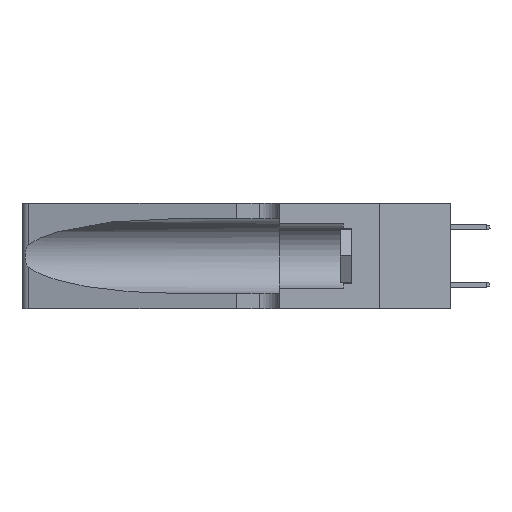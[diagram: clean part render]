
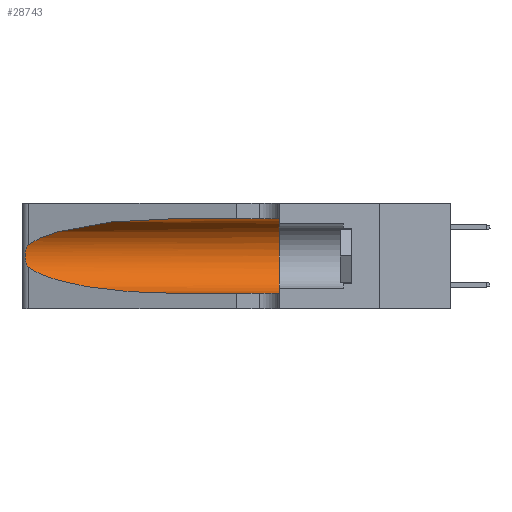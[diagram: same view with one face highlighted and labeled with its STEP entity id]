
A CAD part, left-side view. The second image highlights one B-rep face of the part: STEP entity #28743.
In plain terms, the highlighted cylindrical face has radius 3.308 mm (diameter 6.617 mm), a partial arc.
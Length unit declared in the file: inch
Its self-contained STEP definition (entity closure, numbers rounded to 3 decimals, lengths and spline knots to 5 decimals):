
#1477 = CARTESIAN_POINT ( 'NONE',  ( 0.25854, 1.2359, 0.20912 ) ) ;
#1985 = ORIENTED_EDGE ( 'NONE', *, *, #18966, .F. ) ;
#2399 = VERTEX_POINT ( 'NONE', #12697 ) ;
#2435 = CARTESIAN_POINT ( 'NONE',  ( 0.25487, 1.22718, 0.14631 ) ) ;
#2916 = DIRECTION ( 'NONE',  ( 0., 0., 1. ) ) ;
#3120 = CARTESIAN_POINT ( 'NONE',  ( 0.18966, 0.96281, 0.05475 ) ) ;
#3966 = EDGE_CURVE ( 'NONE', #5168, #22047, #23869, .T. ) ;
#4145 = DIRECTION ( 'NONE',  ( 0., -1., 0. ) ) ;
#5168 = VERTEX_POINT ( 'NONE', #2435 ) ;
#6362 = CARTESIAN_POINT ( 'NONE',  ( 0.18966, 0.96281, 0.31525 ) ) ;
#6592 = CARTESIAN_POINT ( 'NONE',  ( 0.25487, 1.22718, 0.22369 ) ) ;
#6700 = B_SPLINE_CURVE_WITH_KNOTS ( 'NONE', 3,
 ( #29858, #33833, #26591, #15819, #1477, #12050, #41559, #40862, #19999, #26364, #40637, #23302, #19769, #19315 ),
 .UNSPECIFIED., .F., .F.,
 ( 4, 2, 2, 2, 2, 2, 4 ),
 ( 0., 0.00027, 0.00053, 0.00107, 0.0016, 0.00187, 0.00214 ),
 .UNSPECIFIED. ) ;
#7445 = CARTESIAN_POINT ( 'NONE',  ( 0.1305, 1.61858, 0.31525 ) ) ;
#8792 = ORIENTED_EDGE ( 'NONE', *, *, #20589, .T. ) ;
#9802 = CIRCLE ( 'NONE', #37466, 0.13025 ) ;
#10226 = VERTEX_POINT ( 'NONE', #25016 ) ;
#11495 = EDGE_CURVE ( 'NONE', #39197, #2399, #28387, .T. ) ;
#12050 = CARTESIAN_POINT ( 'NONE',  ( 0.26018, 1.23835, 0.19895 ) ) ;
#12697 = CARTESIAN_POINT ( 'NONE',  ( 0.25487, 1.22718, 0.22369 ) ) ;
#13379 = CARTESIAN_POINT ( 'NONE',  ( 0.1305, 0.72297, 0.31525 ) ) ;
#13458 = CARTESIAN_POINT ( 'NONE',  ( 0.1305, 1.61858, 0.185 ) ) ;
#14598 = CARTESIAN_POINT ( 'NONE',  ( 0.1305, 0.72297, 0.05475 ) ) ;
#15301 = ORIENTED_EDGE ( 'NONE', *, *, #45141, .T. ) ;
#15819 = CARTESIAN_POINT ( 'NONE',  ( 0.25787, 1.23484, 0.2124 ) ) ;
#15923 = CARTESIAN_POINT ( 'NONE',  ( 0.1305, 0.35, 0.31525 ) ) ;
#16565 = ORIENTED_EDGE ( 'NONE', *, *, #11495, .T. ) ;
#16692 = ORIENTED_EDGE ( 'NONE', *, *, #3966, .T. ) ;
#17470 = DIRECTION ( 'NONE',  ( 0., 0., -1. ) ) ;
#17496 = ORIENTED_EDGE ( 'NONE', *, *, #27423, .F. ) ;
#18966 = EDGE_CURVE ( 'NONE', #39197, #25622, #22671, .T. ) ;
#19315 = CARTESIAN_POINT ( 'NONE',  ( 0.25487, 1.22718, 0.14631 ) ) ;
#19769 = CARTESIAN_POINT ( 'NONE',  ( 0.25555, 1.22993, 0.14849 ) ) ;
#19999 = CARTESIAN_POINT ( 'NONE',  ( 0.26017, 1.23833, 0.17102 ) ) ;
#20381 = AXIS2_PLACEMENT_3D ( 'NONE', #13458, #27777, #17470 ) ;
#20589 = EDGE_CURVE ( 'NONE', #2399, #5168, #6700, .T. ) ;
#22047 = VERTEX_POINT ( 'NONE', #37639 ) ;
#22671 = LINE ( 'NONE', #7445, #32550 ) ;
#23302 = CARTESIAN_POINT ( 'NONE',  ( 0.25639, 1.23186, 0.15144 ) ) ;
#23869 =( BOUNDED_CURVE ( )  B_SPLINE_CURVE ( 3, ( #25375, #32395, #3120, #14598 ),
 .UNSPECIFIED., .F., .T. ) 
 B_SPLINE_CURVE_WITH_KNOTS ( ( 4, 4 ),
 ( 3.44316, 4.71239 ),
 .UNSPECIFIED. ) 
 CURVE ( )  GEOMETRIC_REPRESENTATION_ITEM ( )  RATIONAL_B_SPLINE_CURVE ( ( 1., 0.87, 0.87, 1. ) ) 
 REPRESENTATION_ITEM ( '' )  );
#24488 = FACE_OUTER_BOUND ( 'NONE', #28070, .T. ) ;
#25016 = CARTESIAN_POINT ( 'NONE',  ( 0.1305, 0.35, 0.05475 ) ) ;
#25375 = CARTESIAN_POINT ( 'NONE',  ( 0.25487, 1.22718, 0.14631 ) ) ;
#25622 = VERTEX_POINT ( 'NONE', #15923 ) ;
#25925 = DIRECTION ( 'NONE',  ( 0., -1., 0. ) ) ;
#26364 = CARTESIAN_POINT ( 'NONE',  ( 0.25856, 1.23593, 0.16098 ) ) ;
#26591 = CARTESIAN_POINT ( 'NONE',  ( 0.25639, 1.23184, 0.21858 ) ) ;
#27021 = CARTESIAN_POINT ( 'NONE',  ( 0.1305, 0.72297, 0.31525 ) ) ;
#27423 = EDGE_CURVE ( 'NONE', #25622, #10226, #9802, .T. ) ;
#27777 = DIRECTION ( 'NONE',  ( 0., -1., 0. ) ) ;
#28070 = EDGE_LOOP ( 'NONE', ( #16565, #8792, #16692, #15301, #17496, #1985 ) ) ;
#28387 =( BOUNDED_CURVE ( )  B_SPLINE_CURVE ( 3, ( #13379, #6362, #45713, #6592 ),
 .UNSPECIFIED., .F., .T. ) 
 B_SPLINE_CURVE_WITH_KNOTS ( ( 4, 4 ),
 ( 1.5708, 2.84003 ),
 .UNSPECIFIED. ) 
 CURVE ( )  GEOMETRIC_REPRESENTATION_ITEM ( )  RATIONAL_B_SPLINE_CURVE ( ( 1., 0.87, 0.87, 1. ) ) 
 REPRESENTATION_ITEM ( '' )  );
#28743 = ADVANCED_FACE ( 'NONE', ( #24488 ), #38755, .F. ) ;
#29199 = LINE ( 'NONE', #29441, #45806 ) ;
#29441 = CARTESIAN_POINT ( 'NONE',  ( 0.1305, 1.61858, 0.05475 ) ) ;
#29858 = CARTESIAN_POINT ( 'NONE',  ( 0.25487, 1.22718, 0.22369 ) ) ;
#32395 = CARTESIAN_POINT ( 'NONE',  ( 0.2373, 1.15595, 0.08982 ) ) ;
#32550 = VECTOR ( 'NONE', #4145, 39.37008 ) ;
#33833 = CARTESIAN_POINT ( 'NONE',  ( 0.25555, 1.22994, 0.2215 ) ) ;
#37466 = AXIS2_PLACEMENT_3D ( 'NONE', #38544, #42075, #2916 ) ;
#37639 = CARTESIAN_POINT ( 'NONE',  ( 0.1305, 0.72297, 0.05475 ) ) ;
#38544 = CARTESIAN_POINT ( 'NONE',  ( 0.1305, 0.35, 0.185 ) ) ;
#38755 = CYLINDRICAL_SURFACE ( 'NONE', #20381, 0.13025 ) ;
#39197 = VERTEX_POINT ( 'NONE', #27021 ) ;
#40637 = CARTESIAN_POINT ( 'NONE',  ( 0.25789, 1.23486, 0.15765 ) ) ;
#40862 = CARTESIAN_POINT ( 'NONE',  ( 0.26075, 1.23896, 0.178 ) ) ;
#41559 = CARTESIAN_POINT ( 'NONE',  ( 0.26075, 1.23896, 0.19203 ) ) ;
#42075 = DIRECTION ( 'NONE',  ( 0., 1., 0. ) ) ;
#45141 = EDGE_CURVE ( 'NONE', #22047, #10226, #29199, .T. ) ;
#45713 = CARTESIAN_POINT ( 'NONE',  ( 0.2373, 1.15595, 0.28018 ) ) ;
#45806 = VECTOR ( 'NONE', #25925, 39.37008 ) ;
